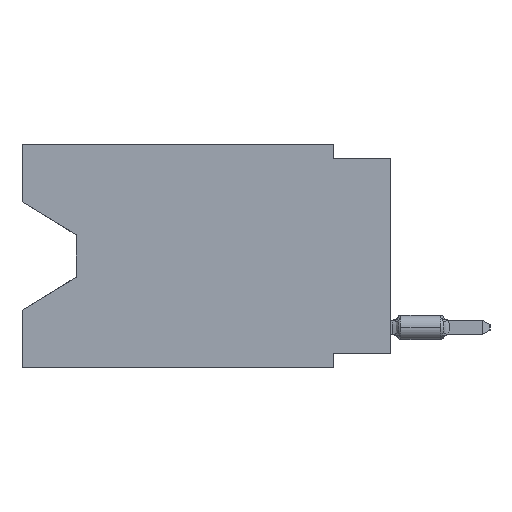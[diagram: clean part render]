
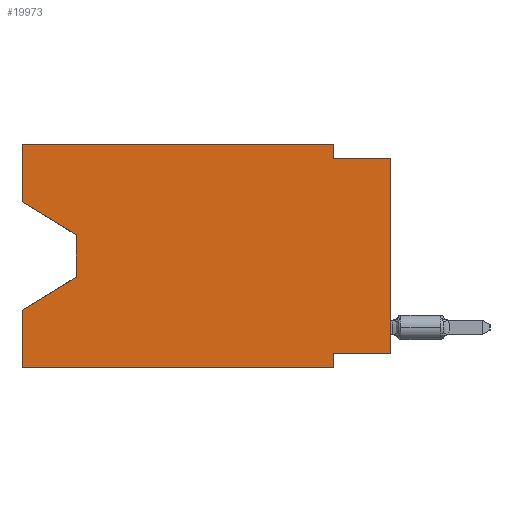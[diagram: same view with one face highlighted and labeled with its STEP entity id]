
A CAD part, left-side view. The second image highlights one B-rep face of the part: STEP entity #19973.
In plain terms, the highlighted planar face has unit normal (-1, 0, 0).
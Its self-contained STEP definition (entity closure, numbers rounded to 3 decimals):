
#986 = LINE ( 'NONE', #32108, #23660 ) ;
#2922 = CARTESIAN_POINT ( 'NONE',  ( 0., 2.54, -9.906 ) ) ;
#3859 = VECTOR ( 'NONE', #20377, 1000. ) ;
#3900 = VERTEX_POINT ( 'NONE', #46356 ) ;
#5994 = VERTEX_POINT ( 'NONE', #25951 ) ;
#6254 = VERTEX_POINT ( 'NONE', #24856 ) ;
#6380 = CARTESIAN_POINT ( 'NONE',  ( 0., 0., -0.635 ) ) ;
#6543 = EDGE_CURVE ( 'NONE', #6254, #62695, #28562, .T. ) ;
#6550 = ORIENTED_EDGE ( 'NONE', *, *, #29594, .F. ) ;
#7116 = EDGE_CURVE ( 'NONE', #5994, #15507, #10738, .T. ) ;
#7423 = CARTESIAN_POINT ( 'NONE',  ( 0., 16.383, 0. ) ) ;
#9322 = CARTESIAN_POINT ( 'NONE',  ( 0., 2.54, 0. ) ) ;
#9520 = AXIS2_PLACEMENT_3D ( 'NONE', #27997, #53959, #53281 ) ;
#9736 = DIRECTION ( 'NONE',  ( 0., 0., 1. ) ) ;
#10738 = LINE ( 'NONE', #20981, #49043 ) ;
#12193 = LINE ( 'NONE', #6380, #41637 ) ;
#12291 = ORIENTED_EDGE ( 'NONE', *, *, #34279, .F. ) ;
#13807 = CARTESIAN_POINT ( 'NONE',  ( 0., 16.383, -7.36 ) ) ;
#15507 = VERTEX_POINT ( 'NONE', #37833 ) ;
#15592 = ORIENTED_EDGE ( 'NONE', *, *, #7116, .T. ) ;
#16048 = DIRECTION ( 'NONE',  ( 0., 1., 0. ) ) ;
#16338 = VERTEX_POINT ( 'NONE', #63910 ) ;
#17083 = PLANE ( 'NONE',  #9520 ) ;
#17256 = VERTEX_POINT ( 'NONE', #13807 ) ;
#17652 = DIRECTION ( 'NONE',  ( 0., -1., 0. ) ) ;
#17772 = LINE ( 'NONE', #33150, #25699 ) ;
#17776 = EDGE_CURVE ( 'NONE', #39258, #17256, #63466, .T. ) ;
#18136 = CARTESIAN_POINT ( 'NONE',  ( 0., 16.383, 0. ) ) ;
#18697 = DIRECTION ( 'NONE',  ( 0., 0., 1. ) ) ;
#18893 = LINE ( 'NONE', #9322, #51204 ) ;
#19215 = DIRECTION ( 'NONE',  ( 0., 0., 1. ) ) ;
#19973 = ADVANCED_FACE ( 'NONE', ( #28343 ), #17083, .F. ) ;
#20377 = DIRECTION ( 'NONE',  ( 0., -0.855, -0.519 ) ) ;
#20508 = EDGE_CURVE ( 'NONE', #29032, #55880, #65160, .T. ) ;
#20981 = CARTESIAN_POINT ( 'NONE',  ( 0., 0., 0. ) ) ;
#22213 = ORIENTED_EDGE ( 'NONE', *, *, #23235, .F. ) ;
#22957 = ORIENTED_EDGE ( 'NONE', *, *, #39336, .F. ) ;
#23235 = EDGE_CURVE ( 'NONE', #16338, #15507, #12193, .T. ) ;
#23255 = LINE ( 'NONE', #33521, #28501 ) ;
#23432 = DIRECTION ( 'NONE',  ( 0., 0., -1. ) ) ;
#23660 = VECTOR ( 'NONE', #16048, 1000. ) ;
#24602 = LINE ( 'NONE', #18136, #59774 ) ;
#24856 = CARTESIAN_POINT ( 'NONE',  ( 0., 2.54, -9.271 ) ) ;
#24861 = VECTOR ( 'NONE', #18697, 1000. ) ;
#25699 = VECTOR ( 'NONE', #38266, 1000. ) ;
#25703 = VECTOR ( 'NONE', #43284, 1000. ) ;
#25951 = CARTESIAN_POINT ( 'NONE',  ( 0., 0., -9.271 ) ) ;
#26660 = CARTESIAN_POINT ( 'NONE',  ( 0., 16.383, -9.906 ) ) ;
#26972 = EDGE_LOOP ( 'NONE', ( #44754, #61470, #65333, #22957, #45949, #52937, #6550, #15592, #22213, #12291, #38444, #59000 ) ) ;
#27997 = CARTESIAN_POINT ( 'NONE',  ( 0., 16.383, 0. ) ) ;
#28343 = FACE_OUTER_BOUND ( 'NONE', #26972, .T. ) ;
#28501 = VECTOR ( 'NONE', #44094, 1000. ) ;
#28562 = LINE ( 'NONE', #2922, #47867 ) ;
#29032 = VERTEX_POINT ( 'NONE', #44944 ) ;
#29594 = EDGE_CURVE ( 'NONE', #5994, #6254, #986, .T. ) ;
#29725 = DIRECTION ( 'NONE',  ( 0., -1., 0. ) ) ;
#31291 = LINE ( 'NONE', #52122, #3859 ) ;
#32108 = CARTESIAN_POINT ( 'NONE',  ( 0., 0., -9.271 ) ) ;
#33150 = CARTESIAN_POINT ( 'NONE',  ( 0., 16.383, -9.906 ) ) ;
#33521 = CARTESIAN_POINT ( 'NONE',  ( 0., 13.97, -4.013 ) ) ;
#34279 = EDGE_CURVE ( 'NONE', #3900, #16338, #18893, .T. ) ;
#37833 = CARTESIAN_POINT ( 'NONE',  ( 0., 0., -0.635 ) ) ;
#38169 = CARTESIAN_POINT ( 'NONE',  ( 0., 13.97, -5.893 ) ) ;
#38266 = DIRECTION ( 'NONE',  ( 0., -1., 0. ) ) ;
#38444 = ORIENTED_EDGE ( 'NONE', *, *, #44406, .F. ) ;
#39258 = VERTEX_POINT ( 'NONE', #67033 ) ;
#39336 = EDGE_CURVE ( 'NONE', #64923, #17256, #55411, .T. ) ;
#41637 = VECTOR ( 'NONE', #17652, 1000. ) ;
#41703 = EDGE_CURVE ( 'NONE', #64923, #62695, #17772, .T. ) ;
#43284 = DIRECTION ( 'NONE',  ( 0., 0.855, -0.519 ) ) ;
#44094 = DIRECTION ( 'NONE',  ( 0., 0., -1. ) ) ;
#44217 = VERTEX_POINT ( 'NONE', #64609 ) ;
#44406 = EDGE_CURVE ( 'NONE', #55880, #3900, #24602, .T. ) ;
#44754 = ORIENTED_EDGE ( 'NONE', *, *, #49113, .T. ) ;
#44944 = CARTESIAN_POINT ( 'NONE',  ( 0., 16.383, -2.546 ) ) ;
#45188 = DIRECTION ( 'NONE',  ( 0., 0., -1. ) ) ;
#45949 = ORIENTED_EDGE ( 'NONE', *, *, #41703, .T. ) ;
#46356 = CARTESIAN_POINT ( 'NONE',  ( 0., 2.54, 0. ) ) ;
#47867 = VECTOR ( 'NONE', #23432, 1000. ) ;
#49043 = VECTOR ( 'NONE', #9736, 1000. ) ;
#49113 = EDGE_CURVE ( 'NONE', #29032, #44217, #31291, .T. ) ;
#51204 = VECTOR ( 'NONE', #45188, 1000. ) ;
#52122 = CARTESIAN_POINT ( 'NONE',  ( 0., 16.383, -2.546 ) ) ;
#52937 = ORIENTED_EDGE ( 'NONE', *, *, #6543, .F. ) ;
#53281 = DIRECTION ( 'NONE',  ( 0., 0., -1. ) ) ;
#53959 = DIRECTION ( 'NONE',  ( 1., 0., 0. ) ) ;
#55411 = LINE ( 'NONE', #66700, #65807 ) ;
#55880 = VERTEX_POINT ( 'NONE', #56931 ) ;
#56895 = EDGE_CURVE ( 'NONE', #44217, #39258, #23255, .T. ) ;
#56931 = CARTESIAN_POINT ( 'NONE',  ( 0., 16.383, 0. ) ) ;
#59000 = ORIENTED_EDGE ( 'NONE', *, *, #20508, .F. ) ;
#59774 = VECTOR ( 'NONE', #29725, 1000. ) ;
#61470 = ORIENTED_EDGE ( 'NONE', *, *, #56895, .T. ) ;
#62695 = VERTEX_POINT ( 'NONE', #66605 ) ;
#63466 = LINE ( 'NONE', #38169, #25703 ) ;
#63910 = CARTESIAN_POINT ( 'NONE',  ( 0., 2.54, -0.635 ) ) ;
#64609 = CARTESIAN_POINT ( 'NONE',  ( 0., 13.97, -4.013 ) ) ;
#64923 = VERTEX_POINT ( 'NONE', #26660 ) ;
#65160 = LINE ( 'NONE', #7423, #24861 ) ;
#65333 = ORIENTED_EDGE ( 'NONE', *, *, #17776, .T. ) ;
#65807 = VECTOR ( 'NONE', #19215, 1000. ) ;
#66605 = CARTESIAN_POINT ( 'NONE',  ( 0., 2.54, -9.906 ) ) ;
#66700 = CARTESIAN_POINT ( 'NONE',  ( 0., 16.383, 0. ) ) ;
#67033 = CARTESIAN_POINT ( 'NONE',  ( 0., 13.97, -5.893 ) ) ;
